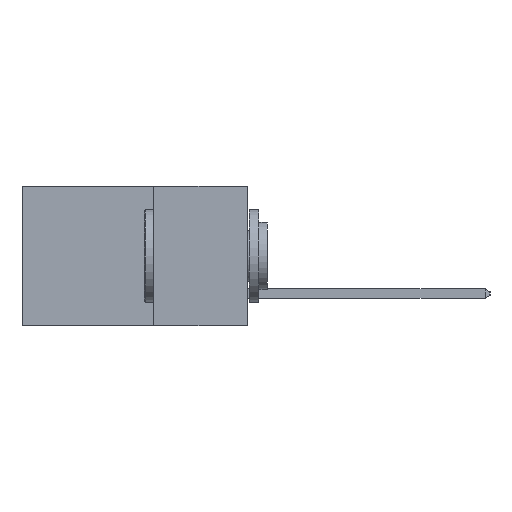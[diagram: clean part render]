
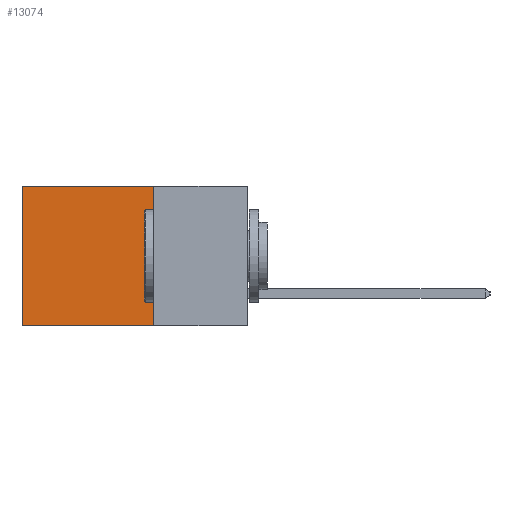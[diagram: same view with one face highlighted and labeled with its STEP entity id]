
A CAD part, left-side view. The second image highlights one B-rep face of the part: STEP entity #13074.
In plain terms, the highlighted planar face has unit normal (-1, 0, 0).
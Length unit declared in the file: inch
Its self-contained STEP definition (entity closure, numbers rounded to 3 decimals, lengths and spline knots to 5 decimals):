
#360 = EDGE_CURVE ( 'NONE', #8662, #10001, #9811, .T. ) ;
#459 = DIRECTION ( 'NONE',  ( 0., 1., 0. ) ) ;
#624 = VERTEX_POINT ( 'NONE', #13037 ) ;
#676 = VECTOR ( 'NONE', #3050, 39.37008 ) ;
#1811 = CARTESIAN_POINT ( 'NONE',  ( 0.2615, 0.25, 0. ) ) ;
#1927 = ORIENTED_EDGE ( 'NONE', *, *, #10187, .F. ) ;
#2103 = DIRECTION ( 'NONE',  ( 0., 0., -1. ) ) ;
#2752 = ORIENTED_EDGE ( 'NONE', *, *, #360, .T. ) ;
#3050 = DIRECTION ( 'NONE',  ( 0., 0., -1. ) ) ;
#3594 = CARTESIAN_POINT ( 'NONE',  ( 0.2615, 0.25, -0.37 ) ) ;
#4566 = DIRECTION ( 'NONE',  ( 1., 0., 0. ) ) ;
#4830 = ORIENTED_EDGE ( 'NONE', *, *, #13851, .T. ) ;
#5056 = VECTOR ( 'NONE', #459, 39.37008 ) ;
#6139 = CARTESIAN_POINT ( 'NONE',  ( 0.2615, 0.25, 0. ) ) ;
#6747 = PLANE ( 'NONE',  #13801 ) ;
#7182 = EDGE_LOOP ( 'NONE', ( #4830, #11736, #1927, #2752 ) ) ;
#8032 = LINE ( 'NONE', #13382, #676 ) ;
#8187 = DIRECTION ( 'NONE',  ( 0., 0., -1. ) ) ;
#8193 = VECTOR ( 'NONE', #14259, 39.37008 ) ;
#8426 = CARTESIAN_POINT ( 'NONE',  ( 0.2615, 0.6, 0. ) ) ;
#8615 = CARTESIAN_POINT ( 'NONE',  ( 0.2615, 0.25, -0.37 ) ) ;
#8662 = VERTEX_POINT ( 'NONE', #6139 ) ;
#9125 = CARTESIAN_POINT ( 'NONE',  ( 0.2615, 0.25, -0.37 ) ) ;
#9811 = LINE ( 'NONE', #1811, #8193 ) ;
#9814 = LINE ( 'NONE', #3594, #9984 ) ;
#9945 = VERTEX_POINT ( 'NONE', #8615 ) ;
#9984 = VECTOR ( 'NONE', #8187, 39.37008 ) ;
#10001 = VERTEX_POINT ( 'NONE', #8426 ) ;
#10187 = EDGE_CURVE ( 'NONE', #8662, #9945, #9814, .T. ) ;
#10793 = LINE ( 'NONE', #12887, #5056 ) ;
#11461 = FACE_OUTER_BOUND ( 'NONE', #7182, .T. ) ;
#11736 = ORIENTED_EDGE ( 'NONE', *, *, #13655, .F. ) ;
#12887 = CARTESIAN_POINT ( 'NONE',  ( 0.2615, 0.25, -0.37 ) ) ;
#13037 = CARTESIAN_POINT ( 'NONE',  ( 0.2615, 0.6, -0.37 ) ) ;
#13074 = ADVANCED_FACE ( 'NONE', ( #11461 ), #6747, .F. ) ;
#13382 = CARTESIAN_POINT ( 'NONE',  ( 0.2615, 0.6, -0.37 ) ) ;
#13655 = EDGE_CURVE ( 'NONE', #9945, #624, #10793, .T. ) ;
#13801 = AXIS2_PLACEMENT_3D ( 'NONE', #9125, #4566, #2103 ) ;
#13851 = EDGE_CURVE ( 'NONE', #10001, #624, #8032, .T. ) ;
#14259 = DIRECTION ( 'NONE',  ( 0., 1., 0. ) ) ;
